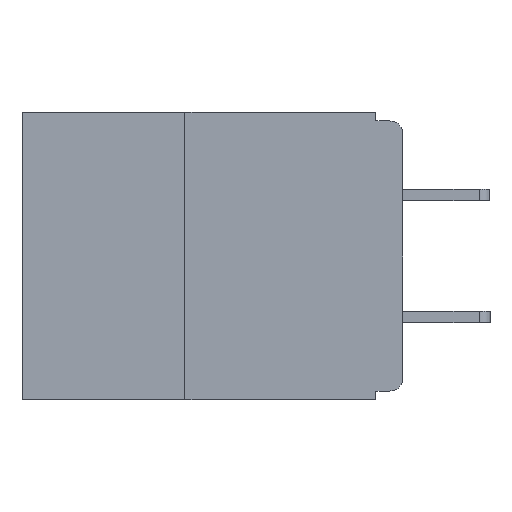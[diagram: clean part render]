
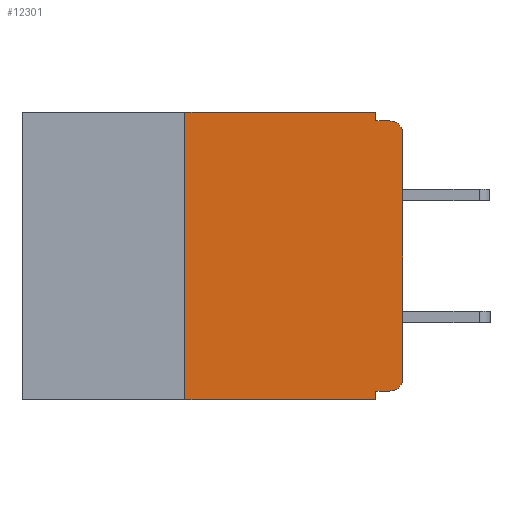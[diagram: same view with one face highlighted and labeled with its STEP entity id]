
A CAD part, left-side view. The second image highlights one B-rep face of the part: STEP entity #12301.
In plain terms, the highlighted planar face has unit normal (-1, 0, 0).
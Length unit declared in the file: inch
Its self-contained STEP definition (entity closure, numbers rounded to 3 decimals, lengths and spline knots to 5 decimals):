
#140 = AXIS2_PLACEMENT_3D ( 'NONE', #3064, #16399, #4981 ) ;
#386 = DIRECTION ( 'NONE',  ( 0., 0., -1. ) ) ;
#607 = CARTESIAN_POINT ( 'NONE',  ( 0., 0.437, -0.33 ) ) ;
#755 = LINE ( 'NONE', #22223, #15953 ) ;
#1038 = CARTESIAN_POINT ( 'NONE',  ( 0., 0.437, 0. ) ) ;
#1835 = EDGE_CURVE ( 'NONE', #11246, #20123, #14412, .T. ) ;
#1916 = LINE ( 'NONE', #16193, #22004 ) ;
#2185 = CARTESIAN_POINT ( 'NONE',  ( 0., 0.015, -0.025 ) ) ;
#2850 = EDGE_CURVE ( 'NONE', #11246, #7858, #12586, .T. ) ;
#2942 = DIRECTION ( 'NONE',  ( 1., 0., 0. ) ) ;
#3064 = CARTESIAN_POINT ( 'NONE',  ( 0., 0.015, -0.305 ) ) ;
#3243 = CARTESIAN_POINT ( 'NONE',  ( 0., 0.031, 0. ) ) ;
#3514 = CARTESIAN_POINT ( 'NONE',  ( 0., 0.015, -0.01 ) ) ;
#4023 = DIRECTION ( 'NONE',  ( 0., -1., 0. ) ) ;
#4131 = DIRECTION ( 'NONE',  ( 0., 0., -1. ) ) ;
#4156 = ORIENTED_EDGE ( 'NONE', *, *, #9094, .T. ) ;
#4787 = PLANE ( 'NONE',  #18508 ) ;
#4861 = CARTESIAN_POINT ( 'NONE',  ( 0., 0.25, -0.33 ) ) ;
#4981 = DIRECTION ( 'NONE',  ( 0., 0., -1. ) ) ;
#5159 = DIRECTION ( 'NONE',  ( 0., 0., -1. ) ) ;
#5477 = VERTEX_POINT ( 'NONE', #3514 ) ;
#5911 = ORIENTED_EDGE ( 'NONE', *, *, #16590, .F. ) ;
#6042 = VECTOR ( 'NONE', #19056, 39.37008 ) ;
#6646 = EDGE_CURVE ( 'NONE', #12610, #18194, #755, .T. ) ;
#6884 = EDGE_CURVE ( 'NONE', #18194, #7858, #24237, .T. ) ;
#7304 = CARTESIAN_POINT ( 'NONE',  ( 0., 0., -0.305 ) ) ;
#7820 = EDGE_LOOP ( 'NONE', ( #9144, #4156, #5911, #18486, #14603, #15235, #14622, #13676, #9938, #14874 ) ) ;
#7858 = VERTEX_POINT ( 'NONE', #16561 ) ;
#8083 = VECTOR ( 'NONE', #19834, 39.37008 ) ;
#9015 = CIRCLE ( 'NONE', #17404, 0.015 ) ;
#9094 = EDGE_CURVE ( 'NONE', #20503, #5477, #9015, .T. ) ;
#9144 = ORIENTED_EDGE ( 'NONE', *, *, #18475, .T. ) ;
#9151 = DIRECTION ( 'NONE',  ( 0., 1., 0. ) ) ;
#9423 = VECTOR ( 'NONE', #386, 39.37008 ) ;
#9938 = ORIENTED_EDGE ( 'NONE', *, *, #6646, .F. ) ;
#9968 = EDGE_CURVE ( 'NONE', #15723, #13573, #10795, .T. ) ;
#10598 = DIRECTION ( 'NONE',  ( 0., -1., 0. ) ) ;
#10795 = LINE ( 'NONE', #3243, #14062 ) ;
#11167 = LINE ( 'NONE', #18977, #6042 ) ;
#11240 = VECTOR ( 'NONE', #4023, 39.37008 ) ;
#11246 = VERTEX_POINT ( 'NONE', #4861 ) ;
#12301 = ADVANCED_FACE ( 'NONE', ( #17745 ), #4787, .F. ) ;
#12586 = LINE ( 'NONE', #607, #8083 ) ;
#12610 = VERTEX_POINT ( 'NONE', #24326 ) ;
#13573 = VERTEX_POINT ( 'NONE', #19912 ) ;
#13676 = ORIENTED_EDGE ( 'NONE', *, *, #6884, .F. ) ;
#13795 = DIRECTION ( 'NONE',  ( 0., 0., 1. ) ) ;
#14062 = VECTOR ( 'NONE', #5159, 39.37008 ) ;
#14412 = LINE ( 'NONE', #15895, #19331 ) ;
#14603 = ORIENTED_EDGE ( 'NONE', *, *, #21049, .F. ) ;
#14622 = ORIENTED_EDGE ( 'NONE', *, *, #2850, .T. ) ;
#14874 = ORIENTED_EDGE ( 'NONE', *, *, #15598, .T. ) ;
#15235 = ORIENTED_EDGE ( 'NONE', *, *, #1835, .F. ) ;
#15430 = CARTESIAN_POINT ( 'NONE',  ( 0., 0., -0.01 ) ) ;
#15537 = DIRECTION ( 'NONE',  ( -1., 0., 0. ) ) ;
#15598 = EDGE_CURVE ( 'NONE', #12610, #22542, #24006, .T. ) ;
#15723 = VERTEX_POINT ( 'NONE', #20242 ) ;
#15895 = CARTESIAN_POINT ( 'NONE',  ( 0., 0.25, -0.33 ) ) ;
#15953 = VECTOR ( 'NONE', #9151, 39.37008 ) ;
#16193 = CARTESIAN_POINT ( 'NONE',  ( 0., 0.437, 0. ) ) ;
#16233 = LINE ( 'NONE', #15430, #11240 ) ;
#16265 = CARTESIAN_POINT ( 'NONE',  ( 0., 0.031, -0.32 ) ) ;
#16286 = DIRECTION ( 'NONE',  ( 0., 0., -1. ) ) ;
#16399 = DIRECTION ( 'NONE',  ( -1., 0., 0. ) ) ;
#16561 = CARTESIAN_POINT ( 'NONE',  ( 0., 0.031, -0.33 ) ) ;
#16590 = EDGE_CURVE ( 'NONE', #13573, #5477, #16233, .T. ) ;
#17404 = AXIS2_PLACEMENT_3D ( 'NONE', #2185, #15537, #4131 ) ;
#17745 = FACE_OUTER_BOUND ( 'NONE', #7820, .T. ) ;
#17924 = CARTESIAN_POINT ( 'NONE',  ( 0., 0., -0.025 ) ) ;
#18194 = VERTEX_POINT ( 'NONE', #16265 ) ;
#18475 = EDGE_CURVE ( 'NONE', #22542, #20503, #11167, .T. ) ;
#18486 = ORIENTED_EDGE ( 'NONE', *, *, #9968, .F. ) ;
#18508 = AXIS2_PLACEMENT_3D ( 'NONE', #1038, #2942, #16286 ) ;
#18977 = CARTESIAN_POINT ( 'NONE',  ( 0., 0., 0. ) ) ;
#19056 = DIRECTION ( 'NONE',  ( 0., 0., 1. ) ) ;
#19331 = VECTOR ( 'NONE', #13795, 39.37008 ) ;
#19834 = DIRECTION ( 'NONE',  ( 0., -1., 0. ) ) ;
#19912 = CARTESIAN_POINT ( 'NONE',  ( 0., 0.031, -0.01 ) ) ;
#20123 = VERTEX_POINT ( 'NONE', #24152 ) ;
#20242 = CARTESIAN_POINT ( 'NONE',  ( 0., 0.031, 0. ) ) ;
#20503 = VERTEX_POINT ( 'NONE', #17924 ) ;
#21049 = EDGE_CURVE ( 'NONE', #20123, #15723, #1916, .T. ) ;
#21102 = CARTESIAN_POINT ( 'NONE',  ( 0., 0.031, -0.33 ) ) ;
#22004 = VECTOR ( 'NONE', #10598, 39.37008 ) ;
#22223 = CARTESIAN_POINT ( 'NONE',  ( 0., 0., -0.32 ) ) ;
#22542 = VERTEX_POINT ( 'NONE', #7304 ) ;
#24006 = CIRCLE ( 'NONE', #140, 0.015 ) ;
#24152 = CARTESIAN_POINT ( 'NONE',  ( 0., 0.25, 0. ) ) ;
#24237 = LINE ( 'NONE', #21102, #9423 ) ;
#24326 = CARTESIAN_POINT ( 'NONE',  ( 0., 0.015, -0.32 ) ) ;
